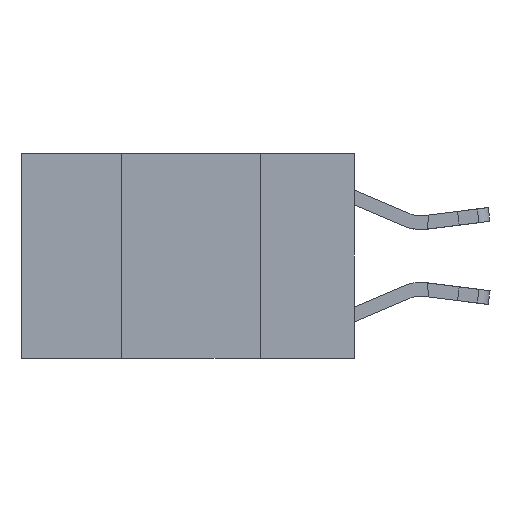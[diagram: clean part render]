
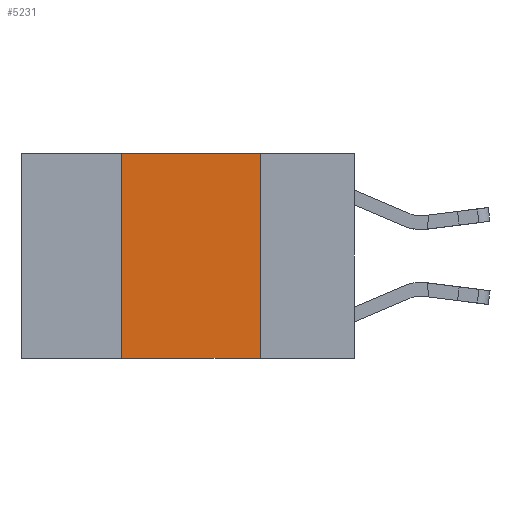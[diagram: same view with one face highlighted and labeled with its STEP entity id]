
A CAD part, left-side view. The second image highlights one B-rep face of the part: STEP entity #5231.
In plain terms, the highlighted planar face has unit normal (-1, 0, 0).
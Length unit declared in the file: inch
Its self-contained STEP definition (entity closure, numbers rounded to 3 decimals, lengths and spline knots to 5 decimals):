
#588 = EDGE_CURVE ( 'NONE', #17454, #3937, #8063, .T. ) ;
#1760 = VERTEX_POINT ( 'NONE', #8976 ) ;
#1811 = VECTOR ( 'NONE', #21536, 39.37008 ) ;
#2081 = AXIS2_PLACEMENT_3D ( 'NONE', #18654, #7916, #20422 ) ;
#2662 = ORIENTED_EDGE ( 'NONE', *, *, #588, .F. ) ;
#2970 = LINE ( 'NONE', #3589, #1811 ) ;
#3028 = ORIENTED_EDGE ( 'NONE', *, *, #13701, .T. ) ;
#3589 = CARTESIAN_POINT ( 'NONE',  ( 0., 0.6, 0. ) ) ;
#3937 = VERTEX_POINT ( 'NONE', #6212 ) ;
#5231 = ADVANCED_FACE ( 'NONE', ( #6701 ), #20347, .F. ) ;
#5455 = VECTOR ( 'NONE', #18009, 39.37008 ) ;
#5673 = EDGE_CURVE ( 'NONE', #1760, #17454, #2970, .T. ) ;
#6078 = DIRECTION ( 'NONE',  ( 0., 0., 1. ) ) ;
#6212 = CARTESIAN_POINT ( 'NONE',  ( 0., 0.17, -0.37 ) ) ;
#6701 = FACE_OUTER_BOUND ( 'NONE', #10268, .T. ) ;
#7496 = VECTOR ( 'NONE', #10969, 39.37008 ) ;
#7916 = DIRECTION ( 'NONE',  ( 1., 0., 0. ) ) ;
#8063 = LINE ( 'NONE', #12403, #7496 ) ;
#8407 = EDGE_CURVE ( 'NONE', #10808, #1760, #15797, .T. ) ;
#8976 = CARTESIAN_POINT ( 'NONE',  ( 0., 0.42, 0. ) ) ;
#10268 = EDGE_LOOP ( 'NONE', ( #2662, #12212, #17484, #3028 ) ) ;
#10808 = VERTEX_POINT ( 'NONE', #12673 ) ;
#10969 = DIRECTION ( 'NONE',  ( 0., 0., -1. ) ) ;
#12212 = ORIENTED_EDGE ( 'NONE', *, *, #5673, .F. ) ;
#12403 = CARTESIAN_POINT ( 'NONE',  ( 0., 0.17, 0. ) ) ;
#12673 = CARTESIAN_POINT ( 'NONE',  ( 0., 0.42, -0.37 ) ) ;
#13701 = EDGE_CURVE ( 'NONE', #10808, #3937, #19765, .T. ) ;
#15035 = CARTESIAN_POINT ( 'NONE',  ( 0., 0.42, 0. ) ) ;
#15797 = LINE ( 'NONE', #15035, #19972 ) ;
#17454 = VERTEX_POINT ( 'NONE', #20762 ) ;
#17484 = ORIENTED_EDGE ( 'NONE', *, *, #8407, .F. ) ;
#18009 = DIRECTION ( 'NONE',  ( 0., -1., 0. ) ) ;
#18654 = CARTESIAN_POINT ( 'NONE',  ( 0., 0.6, 0. ) ) ;
#19765 = LINE ( 'NONE', #21517, #5455 ) ;
#19972 = VECTOR ( 'NONE', #6078, 39.37008 ) ;
#20347 = PLANE ( 'NONE',  #2081 ) ;
#20422 = DIRECTION ( 'NONE',  ( 0., 0., -1. ) ) ;
#20762 = CARTESIAN_POINT ( 'NONE',  ( 0., 0.17, 0. ) ) ;
#21517 = CARTESIAN_POINT ( 'NONE',  ( 0., 0.6, -0.37 ) ) ;
#21536 = DIRECTION ( 'NONE',  ( 0., -1., 0. ) ) ;
